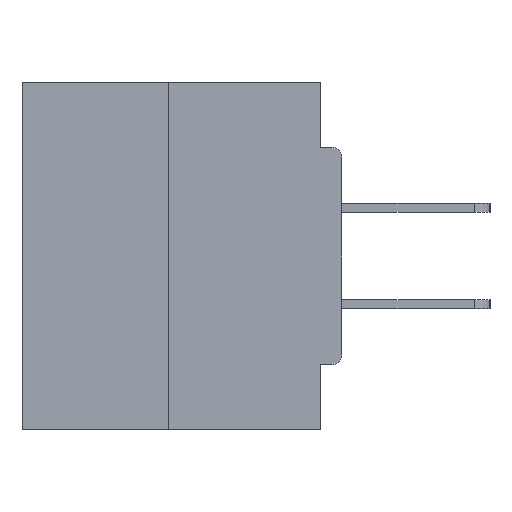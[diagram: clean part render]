
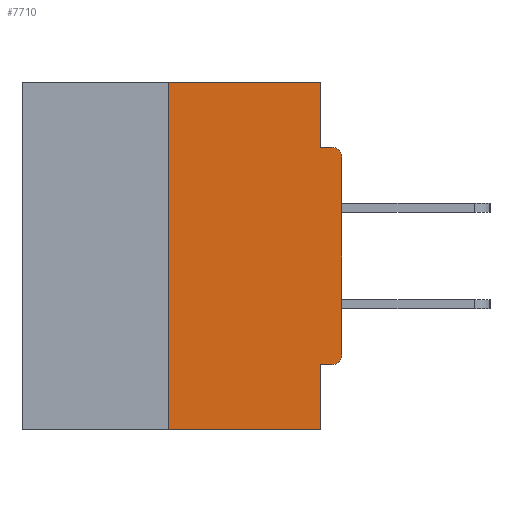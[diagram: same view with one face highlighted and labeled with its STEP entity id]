
A CAD part, left-side view. The second image highlights one B-rep face of the part: STEP entity #7710.
In plain terms, the highlighted planar face has unit normal (-1, 0, 0).
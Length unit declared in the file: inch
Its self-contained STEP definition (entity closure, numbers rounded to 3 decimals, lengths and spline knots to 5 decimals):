
#298 = ORIENTED_EDGE ( 'NONE', *, *, #13687, .F. ) ;
#627 = EDGE_CURVE ( 'NONE', #3231, #24262, #15813, .T. ) ;
#1520 = DIRECTION ( 'NONE',  ( 0., 0., -1. ) ) ;
#2367 = CIRCLE ( 'NONE', #9586, 0.015 ) ;
#3231 = VERTEX_POINT ( 'NONE', #10629 ) ;
#3872 = DIRECTION ( 'NONE',  ( 0., -1., 0. ) ) ;
#4678 = ORIENTED_EDGE ( 'NONE', *, *, #16357, .F. ) ;
#4696 = DIRECTION ( 'NONE',  ( 0., 0., 1. ) ) ;
#5604 = DIRECTION ( 'NONE',  ( 1., 0., 0. ) ) ;
#5689 = LINE ( 'NONE', #8934, #24517 ) ;
#5937 = CARTESIAN_POINT ( 'NONE',  ( 0., 0.46, 0. ) ) ;
#5952 = LINE ( 'NONE', #6107, #17829 ) ;
#6107 = CARTESIAN_POINT ( 'NONE',  ( 0., 0.46, 0. ) ) ;
#6206 = CARTESIAN_POINT ( 'NONE',  ( 0., 0.031, 0. ) ) ;
#6459 = LINE ( 'NONE', #25043, #16240 ) ;
#6972 = EDGE_CURVE ( 'NONE', #16977, #28726, #22025, .T. ) ;
#7017 = ORIENTED_EDGE ( 'NONE', *, *, #19101, .T. ) ;
#7022 = VERTEX_POINT ( 'NONE', #24793 ) ;
#7710 = ADVANCED_FACE ( 'NONE', ( #30184 ), #8344, .F. ) ;
#7721 = DIRECTION ( 'NONE',  ( 0., 0., -1. ) ) ;
#7782 = EDGE_CURVE ( 'NONE', #10210, #24262, #2367, .T. ) ;
#8344 = PLANE ( 'NONE',  #31259 ) ;
#8406 = CARTESIAN_POINT ( 'NONE',  ( 0., 0.031, -0.4065 ) ) ;
#8698 = VERTEX_POINT ( 'NONE', #24621 ) ;
#8934 = CARTESIAN_POINT ( 'NONE',  ( 0., 0.031, -0.5 ) ) ;
#8938 = DIRECTION ( 'NONE',  ( 0., 0., -1. ) ) ;
#9095 = CIRCLE ( 'NONE', #12554, 0.015 ) ;
#9424 = ORIENTED_EDGE ( 'NONE', *, *, #627, .F. ) ;
#9586 = AXIS2_PLACEMENT_3D ( 'NONE', #16314, #21375, #31886 ) ;
#9858 = DIRECTION ( 'NONE',  ( 0., 1., 0. ) ) ;
#9988 = VERTEX_POINT ( 'NONE', #31107 ) ;
#10210 = VERTEX_POINT ( 'NONE', #21078 ) ;
#10358 = ORIENTED_EDGE ( 'NONE', *, *, #18180, .F. ) ;
#10629 = CARTESIAN_POINT ( 'NONE',  ( 0., 0.031, -0.0935 ) ) ;
#12347 = ORIENTED_EDGE ( 'NONE', *, *, #6972, .T. ) ;
#12554 = AXIS2_PLACEMENT_3D ( 'NONE', #12844, #25653, #7721 ) ;
#12844 = CARTESIAN_POINT ( 'NONE',  ( 0., 0.015, -0.3915 ) ) ;
#13687 = EDGE_CURVE ( 'NONE', #26691, #3231, #17599, .T. ) ;
#15813 = LINE ( 'NONE', #22823, #22776 ) ;
#16240 = VECTOR ( 'NONE', #4696, 39.37008 ) ;
#16314 = CARTESIAN_POINT ( 'NONE',  ( 0., 0.015, -0.1085 ) ) ;
#16357 = EDGE_CURVE ( 'NONE', #7022, #16808, #30780, .T. ) ;
#16808 = VERTEX_POINT ( 'NONE', #8406 ) ;
#16892 = CARTESIAN_POINT ( 'NONE',  ( 0., 0.46, -0.5 ) ) ;
#16977 = VERTEX_POINT ( 'NONE', #26776 ) ;
#17227 = EDGE_CURVE ( 'NONE', #16977, #9988, #31929, .T. ) ;
#17599 = LINE ( 'NONE', #6206, #24158 ) ;
#17829 = VECTOR ( 'NONE', #24500, 39.37008 ) ;
#18180 = EDGE_CURVE ( 'NONE', #16808, #28726, #5689, .T. ) ;
#18870 = VECTOR ( 'NONE', #29798, 39.37008 ) ;
#19101 = EDGE_CURVE ( 'NONE', #8698, #10210, #6459, .T. ) ;
#21078 = CARTESIAN_POINT ( 'NONE',  ( 0., 0., -0.1085 ) ) ;
#21375 = DIRECTION ( 'NONE',  ( -1., 0., 0. ) ) ;
#21601 = VECTOR ( 'NONE', #3872, 39.37008 ) ;
#22025 = LINE ( 'NONE', #16892, #21601 ) ;
#22638 = ORIENTED_EDGE ( 'NONE', *, *, #28690, .T. ) ;
#22776 = VECTOR ( 'NONE', #28080, 39.37008 ) ;
#22823 = CARTESIAN_POINT ( 'NONE',  ( 0., 0., -0.0935 ) ) ;
#23347 = CARTESIAN_POINT ( 'NONE',  ( 0., 0., -0.4065 ) ) ;
#23479 = CARTESIAN_POINT ( 'NONE',  ( 0., 0.031, -0.5 ) ) ;
#24158 = VECTOR ( 'NONE', #8938, 39.37008 ) ;
#24262 = VERTEX_POINT ( 'NONE', #31860 ) ;
#24500 = DIRECTION ( 'NONE',  ( 0., -1., 0. ) ) ;
#24517 = VECTOR ( 'NONE', #1520, 39.37008 ) ;
#24621 = CARTESIAN_POINT ( 'NONE',  ( 0., 0., -0.3915 ) ) ;
#24793 = CARTESIAN_POINT ( 'NONE',  ( 0., 0.015, -0.4065 ) ) ;
#25043 = CARTESIAN_POINT ( 'NONE',  ( 0., 0., 0. ) ) ;
#25653 = DIRECTION ( 'NONE',  ( -1., 0., 0. ) ) ;
#26691 = VERTEX_POINT ( 'NONE', #29370 ) ;
#26776 = CARTESIAN_POINT ( 'NONE',  ( 0., 0.25, -0.5 ) ) ;
#27400 = CARTESIAN_POINT ( 'NONE',  ( 0., 0.25, 0. ) ) ;
#28080 = DIRECTION ( 'NONE',  ( 0., -1., 0. ) ) ;
#28690 = EDGE_CURVE ( 'NONE', #7022, #8698, #9095, .T. ) ;
#28726 = VERTEX_POINT ( 'NONE', #23479 ) ;
#28745 = ORIENTED_EDGE ( 'NONE', *, *, #32082, .F. ) ;
#29157 = DIRECTION ( 'NONE',  ( 0., 0., -1. ) ) ;
#29370 = CARTESIAN_POINT ( 'NONE',  ( 0., 0.031, 0. ) ) ;
#29798 = DIRECTION ( 'NONE',  ( 0., 0., 1. ) ) ;
#29932 = EDGE_LOOP ( 'NONE', ( #28745, #33233, #12347, #10358, #4678, #22638, #7017, #32434, #9424, #298 ) ) ;
#30184 = FACE_OUTER_BOUND ( 'NONE', #29932, .T. ) ;
#30780 = LINE ( 'NONE', #23347, #33621 ) ;
#31107 = CARTESIAN_POINT ( 'NONE',  ( 0., 0.25, 0. ) ) ;
#31259 = AXIS2_PLACEMENT_3D ( 'NONE', #5937, #5604, #29157 ) ;
#31860 = CARTESIAN_POINT ( 'NONE',  ( 0., 0.015, -0.0935 ) ) ;
#31886 = DIRECTION ( 'NONE',  ( 0., 0., -1. ) ) ;
#31929 = LINE ( 'NONE', #27400, #18870 ) ;
#32082 = EDGE_CURVE ( 'NONE', #9988, #26691, #5952, .T. ) ;
#32434 = ORIENTED_EDGE ( 'NONE', *, *, #7782, .T. ) ;
#33233 = ORIENTED_EDGE ( 'NONE', *, *, #17227, .F. ) ;
#33621 = VECTOR ( 'NONE', #9858, 39.37008 ) ;
